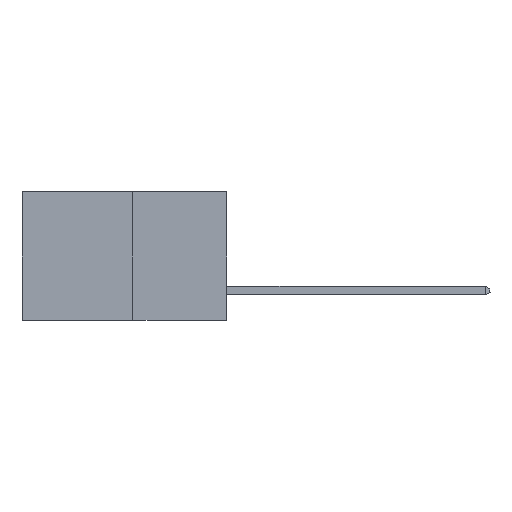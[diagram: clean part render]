
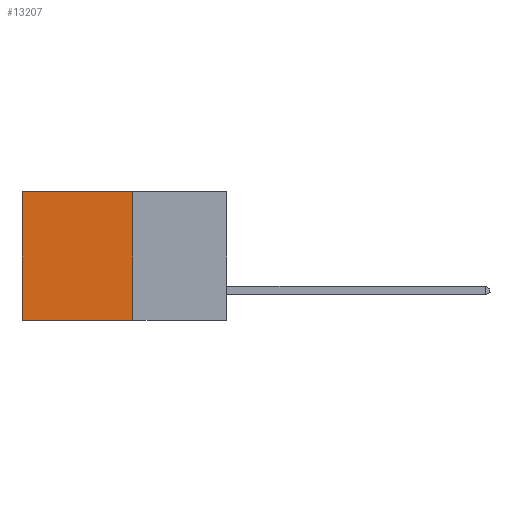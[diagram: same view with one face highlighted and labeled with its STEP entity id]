
A CAD part, left-side view. The second image highlights one B-rep face of the part: STEP entity #13207.
In plain terms, the highlighted planar face has unit normal (-1, 0, 0).
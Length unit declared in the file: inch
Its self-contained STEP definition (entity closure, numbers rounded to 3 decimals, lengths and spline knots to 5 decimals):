
#84 = VERTEX_POINT ( 'NONE', #9656 ) ;
#271 = EDGE_CURVE ( 'NONE', #12707, #12569, #2046, .T. ) ;
#500 = FACE_OUTER_BOUND ( 'NONE', #9333, .T. ) ;
#661 = VERTEX_POINT ( 'NONE', #13201 ) ;
#760 = DIRECTION ( 'NONE',  ( 1., 0., 0. ) ) ;
#2046 = LINE ( 'NONE', #12749, #11795 ) ;
#3536 = ORIENTED_EDGE ( 'NONE', *, *, #4841, .F. ) ;
#3728 = ORIENTED_EDGE ( 'NONE', *, *, #7622, .T. ) ;
#4841 = EDGE_CURVE ( 'NONE', #84, #661, #14612, .T. ) ;
#5620 = PLANE ( 'NONE',  #13978 ) ;
#5641 = CARTESIAN_POINT ( 'NONE',  ( 0.277, 0.59, 0. ) ) ;
#7622 = EDGE_CURVE ( 'NONE', #12569, #661, #15268, .T. ) ;
#8099 = CARTESIAN_POINT ( 'NONE',  ( 0.277, 0.27, -0.37 ) ) ;
#8378 = CARTESIAN_POINT ( 'NONE',  ( 0.277, 0.27, 0. ) ) ;
#8959 = LINE ( 'NONE', #15603, #14645 ) ;
#9075 = DIRECTION ( 'NONE',  ( 0., 0., -1. ) ) ;
#9115 = CARTESIAN_POINT ( 'NONE',  ( 0.277, 0.59, -0.37 ) ) ;
#9311 = DIRECTION ( 'NONE',  ( 0., 0., -1. ) ) ;
#9333 = EDGE_LOOP ( 'NONE', ( #3728, #3536, #12852, #12898 ) ) ;
#9452 = DIRECTION ( 'NONE',  ( 0., 1., 0. ) ) ;
#9599 = DIRECTION ( 'NONE',  ( 0., 0., -1. ) ) ;
#9656 = CARTESIAN_POINT ( 'NONE',  ( 0.277, 0.27, -0.37 ) ) ;
#10976 = EDGE_CURVE ( 'NONE', #12707, #84, #8959, .T. ) ;
#11395 = VECTOR ( 'NONE', #13884, 39.37008 ) ;
#11795 = VECTOR ( 'NONE', #9452, 39.37008 ) ;
#12079 = CARTESIAN_POINT ( 'NONE',  ( 0.277, 0.27, -0.37 ) ) ;
#12081 = VECTOR ( 'NONE', #9075, 39.37008 ) ;
#12569 = VERTEX_POINT ( 'NONE', #5641 ) ;
#12707 = VERTEX_POINT ( 'NONE', #8378 ) ;
#12749 = CARTESIAN_POINT ( 'NONE',  ( 0.277, 0.27, 0. ) ) ;
#12852 = ORIENTED_EDGE ( 'NONE', *, *, #10976, .F. ) ;
#12898 = ORIENTED_EDGE ( 'NONE', *, *, #271, .T. ) ;
#13201 = CARTESIAN_POINT ( 'NONE',  ( 0.277, 0.59, -0.37 ) ) ;
#13207 = ADVANCED_FACE ( 'NONE', ( #500 ), #5620, .F. ) ;
#13884 = DIRECTION ( 'NONE',  ( 0., 1., 0. ) ) ;
#13978 = AXIS2_PLACEMENT_3D ( 'NONE', #8099, #760, #9311 ) ;
#14612 = LINE ( 'NONE', #12079, #11395 ) ;
#14645 = VECTOR ( 'NONE', #9599, 39.37008 ) ;
#15268 = LINE ( 'NONE', #9115, #12081 ) ;
#15603 = CARTESIAN_POINT ( 'NONE',  ( 0.277, 0.27, -0.37 ) ) ;
